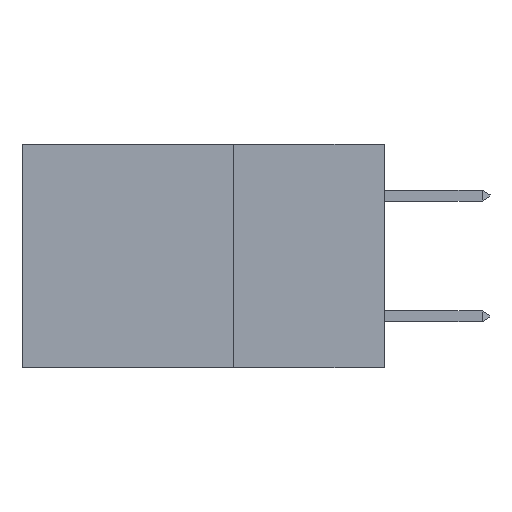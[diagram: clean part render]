
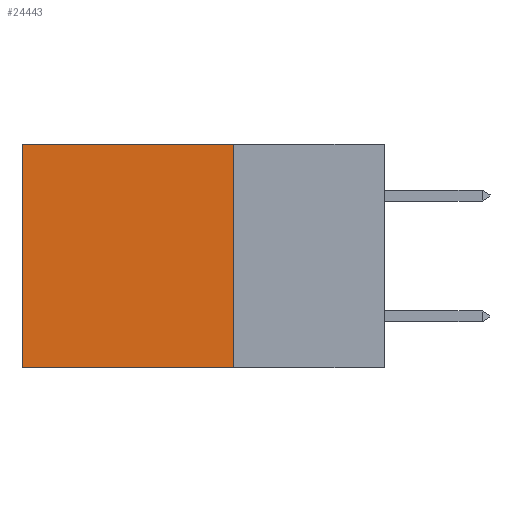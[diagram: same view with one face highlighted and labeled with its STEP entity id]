
A CAD part, left-side view. The second image highlights one B-rep face of the part: STEP entity #24443.
In plain terms, the highlighted planar face has unit normal (-1, 0, 0).
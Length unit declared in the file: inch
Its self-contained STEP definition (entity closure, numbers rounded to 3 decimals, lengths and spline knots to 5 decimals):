
#115 = PLANE ( 'NONE',  #31342 ) ;
#586 = DIRECTION ( 'NONE',  ( 0., 1., 0. ) ) ;
#749 = ORIENTED_EDGE ( 'NONE', *, *, #34428, .T. ) ;
#857 = EDGE_CURVE ( 'NONE', #29613, #6042, #2755, .T. ) ;
#893 = EDGE_CURVE ( 'NONE', #32696, #29613, #37232, .T. ) ;
#1832 = VECTOR ( 'NONE', #2444, 39.37008 ) ;
#2444 = DIRECTION ( 'NONE',  ( 0., 0., -1. ) ) ;
#2755 = LINE ( 'NONE', #14543, #17196 ) ;
#4874 = FACE_OUTER_BOUND ( 'NONE', #27745, .T. ) ;
#5746 = EDGE_CURVE ( 'NONE', #32696, #10602, #16047, .T. ) ;
#6042 = VERTEX_POINT ( 'NONE', #35064 ) ;
#6838 = DIRECTION ( 'NONE',  ( 0., 1., 0. ) ) ;
#8697 = CARTESIAN_POINT ( 'NONE',  ( 0.2875, 0.25, 0. ) ) ;
#10602 = VERTEX_POINT ( 'NONE', #33639 ) ;
#10826 = CARTESIAN_POINT ( 'NONE',  ( 0.2875, 0.6, 0. ) ) ;
#10922 = ORIENTED_EDGE ( 'NONE', *, *, #857, .F. ) ;
#14543 = CARTESIAN_POINT ( 'NONE',  ( 0.2875, 0.25, -0.37 ) ) ;
#16047 = LINE ( 'NONE', #35473, #22857 ) ;
#17196 = VECTOR ( 'NONE', #586, 39.37008 ) ;
#17311 = DIRECTION ( 'NONE',  ( 0., 0., -1. ) ) ;
#22857 = VECTOR ( 'NONE', #6838, 39.37008 ) ;
#23291 = CARTESIAN_POINT ( 'NONE',  ( 0.2875, 0.25, 0. ) ) ;
#24443 = ADVANCED_FACE ( 'NONE', ( #4874 ), #115, .F. ) ;
#25715 = DIRECTION ( 'NONE',  ( 1., 0., 0. ) ) ;
#27745 = EDGE_LOOP ( 'NONE', ( #749, #10922, #36918, #29973 ) ) ;
#28327 = DIRECTION ( 'NONE',  ( 0., 0., -1. ) ) ;
#28768 = CARTESIAN_POINT ( 'NONE',  ( 0.2875, 0.25, 0. ) ) ;
#29613 = VERTEX_POINT ( 'NONE', #36140 ) ;
#29973 = ORIENTED_EDGE ( 'NONE', *, *, #5746, .T. ) ;
#31342 = AXIS2_PLACEMENT_3D ( 'NONE', #8697, #25715, #17311 ) ;
#31409 = LINE ( 'NONE', #10826, #37332 ) ;
#32696 = VERTEX_POINT ( 'NONE', #23291 ) ;
#33639 = CARTESIAN_POINT ( 'NONE',  ( 0.2875, 0.6, 0. ) ) ;
#34428 = EDGE_CURVE ( 'NONE', #10602, #6042, #31409, .T. ) ;
#35064 = CARTESIAN_POINT ( 'NONE',  ( 0.2875, 0.6, -0.37 ) ) ;
#35473 = CARTESIAN_POINT ( 'NONE',  ( 0.2875, 0.25, 0. ) ) ;
#36140 = CARTESIAN_POINT ( 'NONE',  ( 0.2875, 0.25, -0.37 ) ) ;
#36918 = ORIENTED_EDGE ( 'NONE', *, *, #893, .F. ) ;
#37232 = LINE ( 'NONE', #28768, #1832 ) ;
#37332 = VECTOR ( 'NONE', #28327, 39.37008 ) ;
